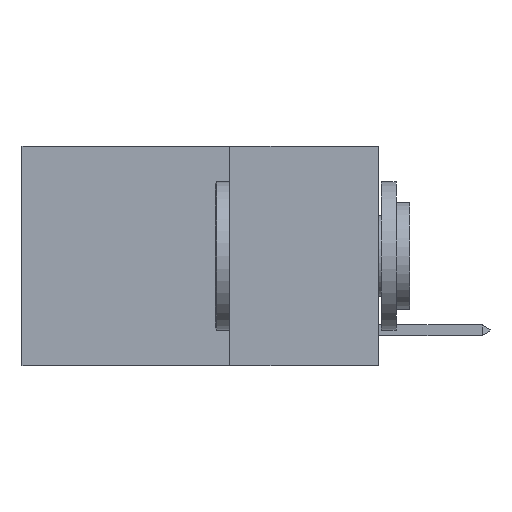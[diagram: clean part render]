
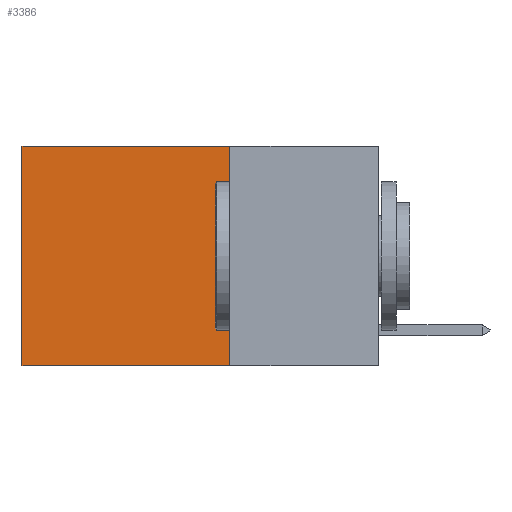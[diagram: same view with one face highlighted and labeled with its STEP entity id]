
A CAD part, left-side view. The second image highlights one B-rep face of the part: STEP entity #3386.
In plain terms, the highlighted planar face has unit normal (-1, 0, 0).
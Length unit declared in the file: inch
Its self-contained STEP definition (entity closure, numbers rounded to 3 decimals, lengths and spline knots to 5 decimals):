
#156 = FACE_OUTER_BOUND ( 'NONE', #5050, .T. ) ;
#306 = VERTEX_POINT ( 'NONE', #4059 ) ;
#569 = CARTESIAN_POINT ( 'NONE',  ( 0.2625, 0.6, 0. ) ) ;
#1368 = VECTOR ( 'NONE', #4708, 39.37008 ) ;
#1705 = VECTOR ( 'NONE', #3177, 39.37008 ) ;
#2027 = PLANE ( 'NONE',  #4550 ) ;
#2372 = LINE ( 'NONE', #569, #10346 ) ;
#2646 = CARTESIAN_POINT ( 'NONE',  ( 0.2625, 0.6, -0.37 ) ) ;
#2995 = EDGE_CURVE ( 'NONE', #306, #11598, #11248, .T. ) ;
#3030 = DIRECTION ( 'NONE',  ( 0., 0., -1. ) ) ;
#3177 = DIRECTION ( 'NONE',  ( 0., 1., 0. ) ) ;
#3241 = CARTESIAN_POINT ( 'NONE',  ( 0.2625, 0.25, -0.37 ) ) ;
#3386 = ADVANCED_FACE ( 'NONE', ( #156 ), #2027, .F. ) ;
#4059 = CARTESIAN_POINT ( 'NONE',  ( 0.2625, 0.25, -0.37 ) ) ;
#4092 = LINE ( 'NONE', #9677, #9242 ) ;
#4147 = EDGE_CURVE ( 'NONE', #9803, #7753, #6668, .T. ) ;
#4550 = AXIS2_PLACEMENT_3D ( 'NONE', #6416, #4756, #6359 ) ;
#4703 = ORIENTED_EDGE ( 'NONE', *, *, #2995, .F. ) ;
#4708 = DIRECTION ( 'NONE',  ( 0., 1., 0. ) ) ;
#4756 = DIRECTION ( 'NONE',  ( 1., 0., 0. ) ) ;
#4853 = CARTESIAN_POINT ( 'NONE',  ( 0.2625, 0.25, 0. ) ) ;
#5050 = EDGE_LOOP ( 'NONE', ( #7297, #4703, #8326, #6847 ) ) ;
#6359 = DIRECTION ( 'NONE',  ( 0., 0., -1. ) ) ;
#6416 = CARTESIAN_POINT ( 'NONE',  ( 0.2625, 0.25, 0. ) ) ;
#6668 = LINE ( 'NONE', #8422, #1368 ) ;
#6847 = ORIENTED_EDGE ( 'NONE', *, *, #4147, .T. ) ;
#6887 = EDGE_CURVE ( 'NONE', #9803, #306, #4092, .T. ) ;
#7297 = ORIENTED_EDGE ( 'NONE', *, *, #8191, .T. ) ;
#7753 = VERTEX_POINT ( 'NONE', #11332 ) ;
#7839 = DIRECTION ( 'NONE',  ( 0., 0., -1. ) ) ;
#8191 = EDGE_CURVE ( 'NONE', #7753, #11598, #2372, .T. ) ;
#8326 = ORIENTED_EDGE ( 'NONE', *, *, #6887, .F. ) ;
#8422 = CARTESIAN_POINT ( 'NONE',  ( 0.2625, 0.25, 0. ) ) ;
#9242 = VECTOR ( 'NONE', #7839, 39.37008 ) ;
#9677 = CARTESIAN_POINT ( 'NONE',  ( 0.2625, 0.25, 0. ) ) ;
#9803 = VERTEX_POINT ( 'NONE', #4853 ) ;
#10346 = VECTOR ( 'NONE', #3030, 39.37008 ) ;
#11248 = LINE ( 'NONE', #3241, #1705 ) ;
#11332 = CARTESIAN_POINT ( 'NONE',  ( 0.2625, 0.6, 0. ) ) ;
#11598 = VERTEX_POINT ( 'NONE', #2646 ) ;
